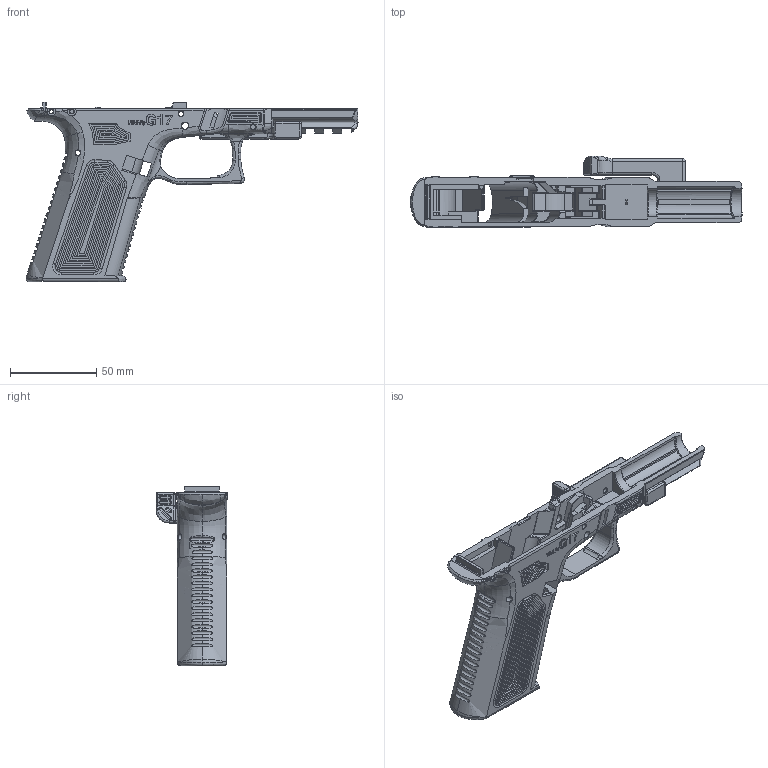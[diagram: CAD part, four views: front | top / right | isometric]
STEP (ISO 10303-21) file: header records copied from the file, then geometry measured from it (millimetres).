
FILE_DESCRIPTION(/* description */ (''),/* implementation_level */ '2;1');
FILE_NAME(/* name */ 'f17-vinh_v1.step',/* time_stamp */ '2020-04-10T04:49:14-04:00',/* author */ (''),/* organization */ (''),/* preprocessor_version */ 'ST-DEVELOPER v18',/* originating_system */ 'Autodesk Translation Framework v8.12.0.6',/* authorisation */ '');
FILE_SCHEMA (('AUTOMOTIVE_DESIGN { 1 0 10303 214 3 1 1 }'));
Products named in the file (3): f17_plainjane; mod10; Thumb Rest
Assembly tree (2 placements, depth 2):
  f17_plainjane
    mod10
    Thumb Rest
Bounding box: 192.61 x 41.68 x 104.43 mm (x, y, z)
Volume: 83325.6 mm3; surface area: 57833.7 mm2
Topology: 3 solids, 3 shells, 1533 faces, 4259 edges, 2756 vertices
Faces by surface type: plane 619, bspline 405, cylinder 389, torus 49, cone 39, sphere 32
Full cylindrical faces by diameter (mm): 2.25 x4, 2.3 x4, 3 x6, 3.091 x27, 4 x30, 7.25 x1
Entity records: 95795 total; most frequent: CARTESIAN_POINT 59517, ORIENTED_EDGE 8460, DIRECTION 6314, EDGE_CURVE 4230, VERTEX_POINT 2756, AXIS2_PLACEMENT_3D 2116, LINE 2082, VECTOR 2082
